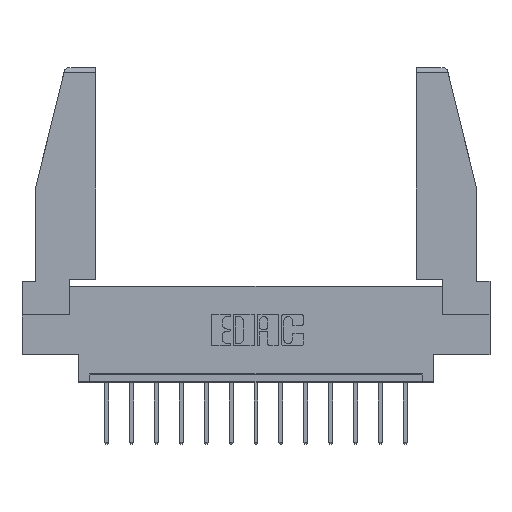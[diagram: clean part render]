
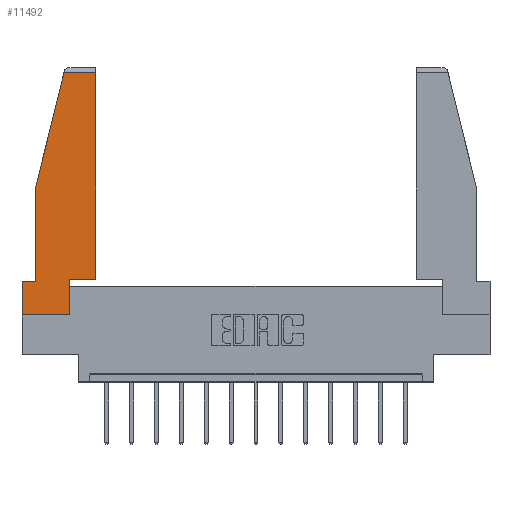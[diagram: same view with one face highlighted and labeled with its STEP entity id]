
A CAD part, top view. The second image highlights one B-rep face of the part: STEP entity #11492.
In plain terms, the highlighted planar face has unit normal (0, 0, 1).
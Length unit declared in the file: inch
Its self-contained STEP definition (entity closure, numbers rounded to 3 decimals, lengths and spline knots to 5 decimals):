
#61 = EDGE_CURVE ( 'NONE', #9769, #2092, #4519, .T. ) ;
#208 = VERTEX_POINT ( 'NONE', #7084 ) ;
#289 = DIRECTION ( 'NONE',  ( 0., 1., 0. ) ) ;
#771 = CARTESIAN_POINT ( 'NONE',  ( 0.086, 0.21, 0. ) ) ;
#1075 = EDGE_CURVE ( 'NONE', #14141, #3176, #14397, .T. ) ;
#1199 = VECTOR ( 'NONE', #15476, 39.37008 ) ;
#1367 = EDGE_CURVE ( 'NONE', #15890, #8327, #12730, .T. ) ;
#1466 = EDGE_CURVE ( 'NONE', #3176, #15890, #5274, .T. ) ;
#1670 = DIRECTION ( 'NONE',  ( 0., 1., 0. ) ) ;
#1816 = CARTESIAN_POINT ( 'NONE',  ( 0., 1.52, 0. ) ) ;
#1931 = VECTOR ( 'NONE', #9870, 39.37008 ) ;
#1970 = LINE ( 'NONE', #7717, #9329 ) ;
#2092 = VERTEX_POINT ( 'NONE', #2461 ) ;
#2304 = ORIENTED_EDGE ( 'NONE', *, *, #1075, .T. ) ;
#2461 = CARTESIAN_POINT ( 'NONE',  ( 0., 0., 0. ) ) ;
#2602 = CARTESIAN_POINT ( 'NONE',  ( 0.271, 1.55, 0. ) ) ;
#2607 = EDGE_CURVE ( 'NONE', #8327, #9769, #15689, .T. ) ;
#2794 = ORIENTED_EDGE ( 'NONE', *, *, #61, .T. ) ;
#3167 = VECTOR ( 'NONE', #15564, 39.37008 ) ;
#3176 = VERTEX_POINT ( 'NONE', #15078 ) ;
#3198 = CARTESIAN_POINT ( 'NONE',  ( 0.086, 0.8, 0. ) ) ;
#3594 = AXIS2_PLACEMENT_3D ( 'NONE', #9607, #11985, #4574 ) ;
#4078 = CARTESIAN_POINT ( 'NONE',  ( 0., 0., 0. ) ) ;
#4519 = LINE ( 'NONE', #12742, #8008 ) ;
#4556 = FACE_OUTER_BOUND ( 'NONE', #14316, .T. ) ;
#4574 = DIRECTION ( 'NONE',  ( 1., 0., 0. ) ) ;
#4879 = VECTOR ( 'NONE', #5109, 39.37008 ) ;
#5084 = CARTESIAN_POINT ( 'NONE',  ( 0.297, 0., 0. ) ) ;
#5109 = DIRECTION ( 'NONE',  ( -0.239, -0.971, 0. ) ) ;
#5274 = LINE ( 'NONE', #2602, #4879 ) ;
#5335 = DIRECTION ( 'NONE',  ( 1., 0., 0. ) ) ;
#5449 = CARTESIAN_POINT ( 'NONE',  ( 0.297, 0., 0. ) ) ;
#5805 = LINE ( 'NONE', #4078, #9853 ) ;
#5990 = PLANE ( 'NONE',  #3594 ) ;
#7006 = ORIENTED_EDGE ( 'NONE', *, *, #1367, .T. ) ;
#7084 = CARTESIAN_POINT ( 'NONE',  ( 0.297, 0.223, 0. ) ) ;
#7717 = CARTESIAN_POINT ( 'NONE',  ( 0.461, 0.223, 0. ) ) ;
#8008 = VECTOR ( 'NONE', #9016, 39.37008 ) ;
#8327 = VERTEX_POINT ( 'NONE', #771 ) ;
#8751 = LINE ( 'NONE', #15524, #1199 ) ;
#9016 = DIRECTION ( 'NONE',  ( 0., -1., 0. ) ) ;
#9052 = VECTOR ( 'NONE', #12902, 39.37008 ) ;
#9105 = ORIENTED_EDGE ( 'NONE', *, *, #2607, .T. ) ;
#9298 = EDGE_CURVE ( 'NONE', #2092, #14223, #5805, .T. ) ;
#9329 = VECTOR ( 'NONE', #289, 39.37008 ) ;
#9397 = ORIENTED_EDGE ( 'NONE', *, *, #13269, .T. ) ;
#9607 = CARTESIAN_POINT ( 'NONE',  ( 0., 0., 0. ) ) ;
#9769 = VERTEX_POINT ( 'NONE', #10831 ) ;
#9853 = VECTOR ( 'NONE', #5335, 39.37008 ) ;
#9870 = DIRECTION ( 'NONE',  ( -1., 0., 0. ) ) ;
#10430 = EDGE_CURVE ( 'NONE', #14223, #208, #12133, .T. ) ;
#10831 = CARTESIAN_POINT ( 'NONE',  ( 0., 0.21, 0. ) ) ;
#10905 = CARTESIAN_POINT ( 'NONE',  ( 0.461, 0.223, 0. ) ) ;
#11131 = CARTESIAN_POINT ( 'NONE',  ( 0., 0.21, 0. ) ) ;
#11492 = ADVANCED_FACE ( 'NONE', ( #4556 ), #5990, .T. ) ;
#11597 = ORIENTED_EDGE ( 'NONE', *, *, #10430, .T. ) ;
#11930 = ORIENTED_EDGE ( 'NONE', *, *, #1466, .T. ) ;
#11985 = DIRECTION ( 'NONE',  ( 0., 0., 1. ) ) ;
#12133 = LINE ( 'NONE', #5449, #13292 ) ;
#12375 = CARTESIAN_POINT ( 'NONE',  ( 0.461, 1.52, 0. ) ) ;
#12381 = VERTEX_POINT ( 'NONE', #10905 ) ;
#12730 = LINE ( 'NONE', #3198, #9052 ) ;
#12742 = CARTESIAN_POINT ( 'NONE',  ( 0., 0.21, 0. ) ) ;
#12902 = DIRECTION ( 'NONE',  ( 0., -1., 0. ) ) ;
#13254 = CARTESIAN_POINT ( 'NONE',  ( 0.086, 0.8, 0. ) ) ;
#13269 = EDGE_CURVE ( 'NONE', #12381, #14141, #1970, .T. ) ;
#13292 = VECTOR ( 'NONE', #1670, 39.37008 ) ;
#13586 = ORIENTED_EDGE ( 'NONE', *, *, #13980, .T. ) ;
#13980 = EDGE_CURVE ( 'NONE', #208, #12381, #8751, .T. ) ;
#14141 = VERTEX_POINT ( 'NONE', #12375 ) ;
#14223 = VERTEX_POINT ( 'NONE', #5084 ) ;
#14316 = EDGE_LOOP ( 'NONE', ( #9397, #2304, #11930, #7006, #9105, #2794, #15175, #11597, #13586 ) ) ;
#14397 = LINE ( 'NONE', #1816, #3167 ) ;
#15078 = CARTESIAN_POINT ( 'NONE',  ( 0.2636, 1.52, 0. ) ) ;
#15175 = ORIENTED_EDGE ( 'NONE', *, *, #9298, .T. ) ;
#15476 = DIRECTION ( 'NONE',  ( 1., 0., 0. ) ) ;
#15524 = CARTESIAN_POINT ( 'NONE',  ( 0.297, 0.223, 0. ) ) ;
#15564 = DIRECTION ( 'NONE',  ( -1., 0., 0. ) ) ;
#15689 = LINE ( 'NONE', #11131, #1931 ) ;
#15890 = VERTEX_POINT ( 'NONE', #13254 ) ;
